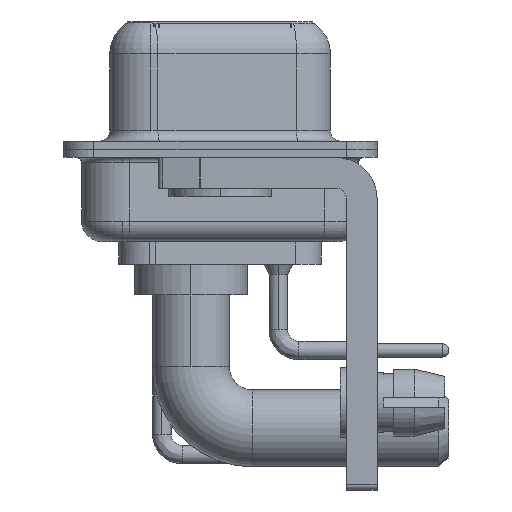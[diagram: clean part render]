
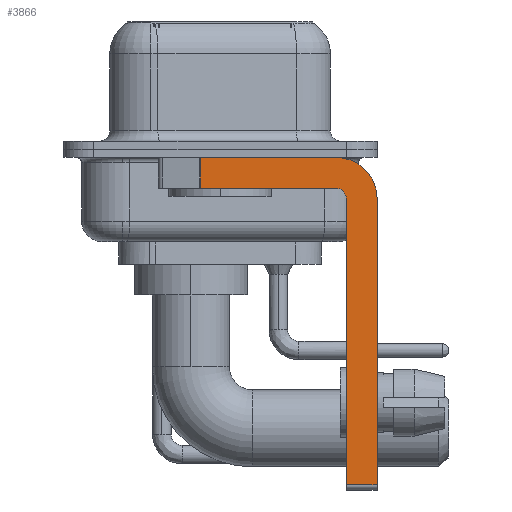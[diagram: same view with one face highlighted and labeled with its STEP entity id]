
A CAD part, left-side view. The second image highlights one B-rep face of the part: STEP entity #3866.
In plain terms, the highlighted planar face has unit normal (-1, 0, 0).
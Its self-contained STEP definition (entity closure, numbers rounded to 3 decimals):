
#748 = DIRECTION ( 'NONE',  ( 0., 0., -1. ) ) ;
#750 = CARTESIAN_POINT ( 'NONE',  ( -2.9, -6.15, -2.4 ) ) ;
#1826 = CARTESIAN_POINT ( 'NONE',  ( -2.9, -5.65, -2.4 ) ) ;
#1830 = VERTEX_POINT ( 'NONE', #31374 ) ;
#2022 = VECTOR ( 'NONE', #29705, 1000. ) ;
#2092 = VECTOR ( 'NONE', #31002, 1000. ) ;
#2403 = EDGE_LOOP ( 'NONE', ( #5747, #13136, #28705, #13276, #27805, #34007, #8588, #28283 ) ) ;
#3866 = ADVANCED_FACE ( 'NONE', ( #15060 ), #23008, .F. ) ;
#3928 = LINE ( 'NONE', #4105, #22964 ) ;
#3987 = CARTESIAN_POINT ( 'NONE',  ( -2.9, -6.15, -16.6 ) ) ;
#4046 = VECTOR ( 'NONE', #19251, 1000. ) ;
#4105 = CARTESIAN_POINT ( 'NONE',  ( -2.9, -5.65, -1.9 ) ) ;
#4451 = CIRCLE ( 'NONE', #19692, 2. ) ;
#5747 = ORIENTED_EDGE ( 'NONE', *, *, #28377, .F. ) ;
#6747 = DIRECTION ( 'NONE',  ( 0., 1., 0. ) ) ;
#7750 = CARTESIAN_POINT ( 'NONE',  ( -2.9, -7.65, -2.4 ) ) ;
#8313 = AXIS2_PLACEMENT_3D ( 'NONE', #23164, #33941, #9744 ) ;
#8588 = ORIENTED_EDGE ( 'NONE', *, *, #32981, .F. ) ;
#9289 = CARTESIAN_POINT ( 'NONE',  ( -2.9, -6.15, -16.35 ) ) ;
#9613 = EDGE_CURVE ( 'NONE', #1830, #31516, #10307, .T. ) ;
#9744 = DIRECTION ( 'NONE',  ( 0., 0., 1. ) ) ;
#10307 = LINE ( 'NONE', #10653, #2022 ) ;
#10653 = CARTESIAN_POINT ( 'NONE',  ( -2.9, 0.978, -1.9 ) ) ;
#13136 = ORIENTED_EDGE ( 'NONE', *, *, #9613, .T. ) ;
#13276 = ORIENTED_EDGE ( 'NONE', *, *, #29171, .F. ) ;
#13537 = CARTESIAN_POINT ( 'NONE',  ( -2.9, -7.65, -2.4 ) ) ;
#13978 = EDGE_CURVE ( 'NONE', #14996, #28887, #22707, .T. ) ;
#14282 = EDGE_CURVE ( 'NONE', #24366, #31516, #3928, .T. ) ;
#14996 = VERTEX_POINT ( 'NONE', #9289 ) ;
#15001 = CARTESIAN_POINT ( 'NONE',  ( -2.9, 0.978, -1.9 ) ) ;
#15060 = FACE_OUTER_BOUND ( 'NONE', #2403, .T. ) ;
#15581 = VERTEX_POINT ( 'NONE', #20725 ) ;
#16063 = LINE ( 'NONE', #26822, #4046 ) ;
#16362 = CARTESIAN_POINT ( 'NONE',  ( -2.9, 3., -0.4 ) ) ;
#17249 = EDGE_CURVE ( 'NONE', #15581, #33452, #4451, .T. ) ;
#19251 = DIRECTION ( 'NONE',  ( 0., -1., 0. ) ) ;
#19692 = AXIS2_PLACEMENT_3D ( 'NONE', #20165, #25457, #748 ) ;
#20165 = CARTESIAN_POINT ( 'NONE',  ( -2.9, -5.65, -2.4 ) ) ;
#20199 = VECTOR ( 'NONE', #28423, 1000. ) ;
#20365 = DIRECTION ( 'NONE',  ( 1., 0., 0. ) ) ;
#20725 = CARTESIAN_POINT ( 'NONE',  ( -2.9, -5.65, -0.4 ) ) ;
#21439 = EDGE_CURVE ( 'NONE', #14996, #30045, #16063, .T. ) ;
#22482 = DIRECTION ( 'NONE',  ( 0., 0., -1. ) ) ;
#22707 = LINE ( 'NONE', #3987, #2092 ) ;
#22964 = VECTOR ( 'NONE', #6747, 1000. ) ;
#23008 = PLANE ( 'NONE',  #31607 ) ;
#23164 = CARTESIAN_POINT ( 'NONE',  ( -2.9, -5.65, -2.4 ) ) ;
#23473 = VECTOR ( 'NONE', #30275, 1000. ) ;
#23826 = LINE ( 'NONE', #7750, #20199 ) ;
#23951 = CARTESIAN_POINT ( 'NONE',  ( -2.9, -5.65, -1.9 ) ) ;
#24298 = CARTESIAN_POINT ( 'NONE',  ( -2.9, -7.65, -16.35 ) ) ;
#24366 = VERTEX_POINT ( 'NONE', #23951 ) ;
#24980 = LINE ( 'NONE', #16362, #23473 ) ;
#25457 = DIRECTION ( 'NONE',  ( 1., 0., 0. ) ) ;
#26822 = CARTESIAN_POINT ( 'NONE',  ( -2.9, -5.65, -16.35 ) ) ;
#27805 = ORIENTED_EDGE ( 'NONE', *, *, #13978, .F. ) ;
#28283 = ORIENTED_EDGE ( 'NONE', *, *, #17249, .F. ) ;
#28377 = EDGE_CURVE ( 'NONE', #1830, #15581, #24980, .T. ) ;
#28423 = DIRECTION ( 'NONE',  ( 0., 0., -1. ) ) ;
#28705 = ORIENTED_EDGE ( 'NONE', *, *, #14282, .F. ) ;
#28887 = VERTEX_POINT ( 'NONE', #750 ) ;
#29171 = EDGE_CURVE ( 'NONE', #28887, #24366, #32564, .T. ) ;
#29705 = DIRECTION ( 'NONE',  ( 0., 0., -1. ) ) ;
#30045 = VERTEX_POINT ( 'NONE', #24298 ) ;
#30275 = DIRECTION ( 'NONE',  ( 0., -1., 0. ) ) ;
#31002 = DIRECTION ( 'NONE',  ( 0., 0., 1. ) ) ;
#31374 = CARTESIAN_POINT ( 'NONE',  ( -2.9, 0.978, -0.4 ) ) ;
#31516 = VERTEX_POINT ( 'NONE', #15001 ) ;
#31607 = AXIS2_PLACEMENT_3D ( 'NONE', #1826, #20365, #22482 ) ;
#32564 = CIRCLE ( 'NONE', #8313, 0.5 ) ;
#32981 = EDGE_CURVE ( 'NONE', #33452, #30045, #23826, .T. ) ;
#33452 = VERTEX_POINT ( 'NONE', #13537 ) ;
#33941 = DIRECTION ( 'NONE',  ( -1., 0., 0. ) ) ;
#34007 = ORIENTED_EDGE ( 'NONE', *, *, #21439, .T. ) ;
